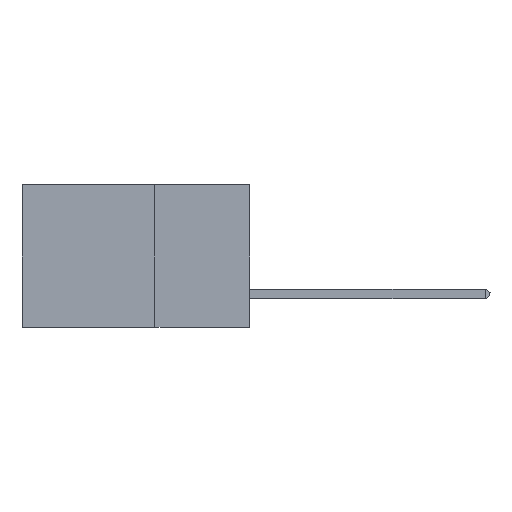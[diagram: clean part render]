
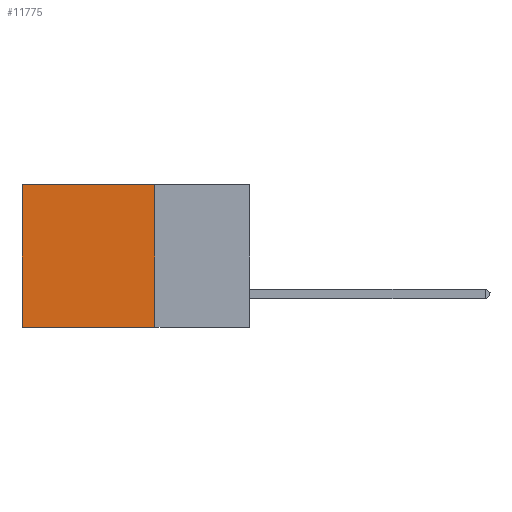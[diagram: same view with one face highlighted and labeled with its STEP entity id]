
A CAD part, left-side view. The second image highlights one B-rep face of the part: STEP entity #11775.
In plain terms, the highlighted planar face has unit normal (-1, 0, 0).
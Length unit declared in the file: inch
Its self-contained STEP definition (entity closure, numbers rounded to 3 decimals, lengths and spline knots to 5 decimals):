
#623 = LINE ( 'NONE', #3935, #8638 ) ;
#635 = EDGE_CURVE ( 'NONE', #3705, #17604, #623, .T. ) ;
#1042 = LINE ( 'NONE', #1515, #4933 ) ;
#1425 = CARTESIAN_POINT ( 'NONE',  ( 0.2875, 0.25, -0.375 ) ) ;
#1515 = CARTESIAN_POINT ( 'NONE',  ( 0.2875, 0.6, -0.375 ) ) ;
#1965 = VECTOR ( 'NONE', #4169, 39.37008 ) ;
#2276 = EDGE_LOOP ( 'NONE', ( #15770, #7472, #16579, #10050 ) ) ;
#2455 = CARTESIAN_POINT ( 'NONE',  ( 0.2875, 0.25, -0.375 ) ) ;
#2798 = DIRECTION ( 'NONE',  ( 0., 0., -1. ) ) ;
#3114 = CARTESIAN_POINT ( 'NONE',  ( 0.2875, 0.6, 0. ) ) ;
#3611 = AXIS2_PLACEMENT_3D ( 'NONE', #5880, #17028, #15624 ) ;
#3705 = VERTEX_POINT ( 'NONE', #10285 ) ;
#3935 = CARTESIAN_POINT ( 'NONE',  ( 0.2875, 0.25, 0. ) ) ;
#4160 = DIRECTION ( 'NONE',  ( 0., 0., -1. ) ) ;
#4169 = DIRECTION ( 'NONE',  ( 0., 1., 0. ) ) ;
#4358 = FACE_OUTER_BOUND ( 'NONE', #2276, .T. ) ;
#4608 = VERTEX_POINT ( 'NONE', #11590 ) ;
#4915 = VERTEX_POINT ( 'NONE', #2455 ) ;
#4933 = VECTOR ( 'NONE', #4160, 39.37008 ) ;
#5880 = CARTESIAN_POINT ( 'NONE',  ( 0.2875, 0.25, -0.375 ) ) ;
#6846 = CARTESIAN_POINT ( 'NONE',  ( 0.2875, 0.25, -0.375 ) ) ;
#7472 = ORIENTED_EDGE ( 'NONE', *, *, #7517, .F. ) ;
#7517 = EDGE_CURVE ( 'NONE', #4915, #4608, #12396, .T. ) ;
#8638 = VECTOR ( 'NONE', #13682, 39.37008 ) ;
#8670 = EDGE_CURVE ( 'NONE', #17604, #4608, #1042, .T. ) ;
#10050 = ORIENTED_EDGE ( 'NONE', *, *, #635, .T. ) ;
#10285 = CARTESIAN_POINT ( 'NONE',  ( 0.2875, 0.25, 0. ) ) ;
#11590 = CARTESIAN_POINT ( 'NONE',  ( 0.2875, 0.6, -0.375 ) ) ;
#11775 = ADVANCED_FACE ( 'NONE', ( #4358 ), #12812, .F. ) ;
#12396 = LINE ( 'NONE', #6846, #1965 ) ;
#12812 = PLANE ( 'NONE',  #3611 ) ;
#12884 = LINE ( 'NONE', #1425, #17034 ) ;
#13682 = DIRECTION ( 'NONE',  ( 0., 1., 0. ) ) ;
#15002 = EDGE_CURVE ( 'NONE', #3705, #4915, #12884, .T. ) ;
#15624 = DIRECTION ( 'NONE',  ( 0., 0., -1. ) ) ;
#15770 = ORIENTED_EDGE ( 'NONE', *, *, #8670, .T. ) ;
#16579 = ORIENTED_EDGE ( 'NONE', *, *, #15002, .F. ) ;
#17028 = DIRECTION ( 'NONE',  ( 1., 0., 0. ) ) ;
#17034 = VECTOR ( 'NONE', #2798, 39.37008 ) ;
#17604 = VERTEX_POINT ( 'NONE', #3114 ) ;
